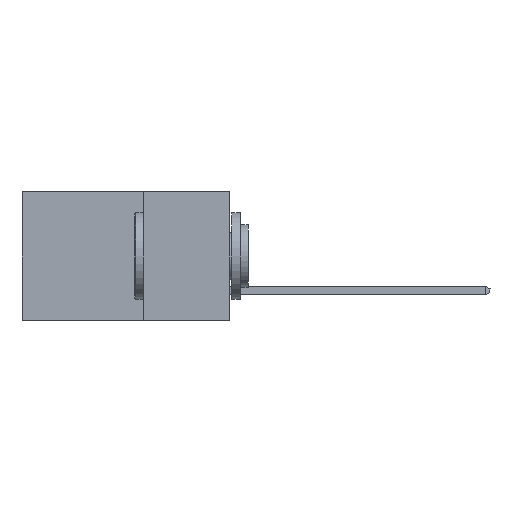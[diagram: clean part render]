
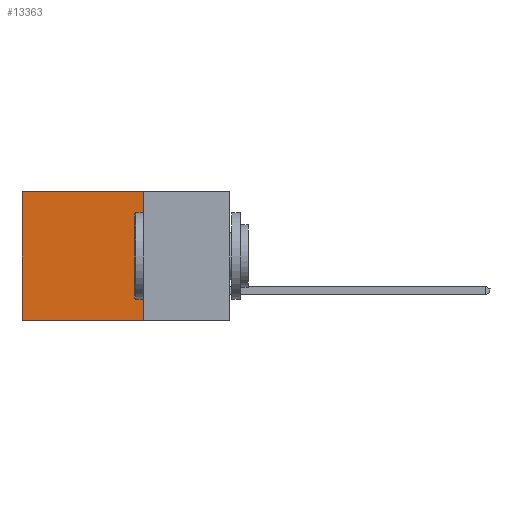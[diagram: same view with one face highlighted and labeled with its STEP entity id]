
A CAD part, left-side view. The second image highlights one B-rep face of the part: STEP entity #13363.
In plain terms, the highlighted planar face has unit normal (-1, 0, 0).
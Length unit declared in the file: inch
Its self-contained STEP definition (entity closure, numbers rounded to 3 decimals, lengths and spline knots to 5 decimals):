
#859 = EDGE_LOOP ( 'NONE', ( #17553, #979, #16050, #10044 ) ) ;
#979 = ORIENTED_EDGE ( 'NONE', *, *, #9617, .F. ) ;
#1090 = VECTOR ( 'NONE', #8352, 39.37008 ) ;
#1432 = AXIS2_PLACEMENT_3D ( 'NONE', #6726, #17992, #14743 ) ;
#1871 = LINE ( 'NONE', #15808, #14584 ) ;
#4482 = EDGE_CURVE ( 'NONE', #7078, #13401, #13876, .T. ) ;
#5580 = LINE ( 'NONE', #7067, #10946 ) ;
#6726 = CARTESIAN_POINT ( 'NONE',  ( 0.2615, 0.25, -0.37 ) ) ;
#7067 = CARTESIAN_POINT ( 'NONE',  ( 0.2615, 0.25, 0. ) ) ;
#7078 = VERTEX_POINT ( 'NONE', #15760 ) ;
#8266 = CARTESIAN_POINT ( 'NONE',  ( 0.2615, 0.25, -0.37 ) ) ;
#8352 = DIRECTION ( 'NONE',  ( 0., 0., -1. ) ) ;
#8363 = LINE ( 'NONE', #13885, #9625 ) ;
#8746 = CARTESIAN_POINT ( 'NONE',  ( 0.2615, 0.25, 0. ) ) ;
#9149 = PLANE ( 'NONE',  #1432 ) ;
#9617 = EDGE_CURVE ( 'NONE', #16375, #13401, #1871, .T. ) ;
#9625 = VECTOR ( 'NONE', #11056, 39.37008 ) ;
#9696 = CARTESIAN_POINT ( 'NONE',  ( 0.2615, 0.6, -0.37 ) ) ;
#10044 = ORIENTED_EDGE ( 'NONE', *, *, #15229, .T. ) ;
#10293 = EDGE_CURVE ( 'NONE', #16352, #16375, #8363, .T. ) ;
#10946 = VECTOR ( 'NONE', #13961, 39.37008 ) ;
#11056 = DIRECTION ( 'NONE',  ( 0., 0., -1. ) ) ;
#13363 = ADVANCED_FACE ( 'NONE', ( #16253 ), #9149, .F. ) ;
#13401 = VERTEX_POINT ( 'NONE', #9696 ) ;
#13876 = LINE ( 'NONE', #16757, #1090 ) ;
#13885 = CARTESIAN_POINT ( 'NONE',  ( 0.2615, 0.25, -0.37 ) ) ;
#13961 = DIRECTION ( 'NONE',  ( 0., 1., 0. ) ) ;
#14584 = VECTOR ( 'NONE', #17188, 39.37008 ) ;
#14743 = DIRECTION ( 'NONE',  ( 0., 0., -1. ) ) ;
#15229 = EDGE_CURVE ( 'NONE', #16352, #7078, #5580, .T. ) ;
#15760 = CARTESIAN_POINT ( 'NONE',  ( 0.2615, 0.6, 0. ) ) ;
#15808 = CARTESIAN_POINT ( 'NONE',  ( 0.2615, 0.25, -0.37 ) ) ;
#16050 = ORIENTED_EDGE ( 'NONE', *, *, #10293, .F. ) ;
#16253 = FACE_OUTER_BOUND ( 'NONE', #859, .T. ) ;
#16352 = VERTEX_POINT ( 'NONE', #8746 ) ;
#16375 = VERTEX_POINT ( 'NONE', #8266 ) ;
#16757 = CARTESIAN_POINT ( 'NONE',  ( 0.2615, 0.6, -0.37 ) ) ;
#17188 = DIRECTION ( 'NONE',  ( 0., 1., 0. ) ) ;
#17553 = ORIENTED_EDGE ( 'NONE', *, *, #4482, .T. ) ;
#17992 = DIRECTION ( 'NONE',  ( 1., 0., 0. ) ) ;
